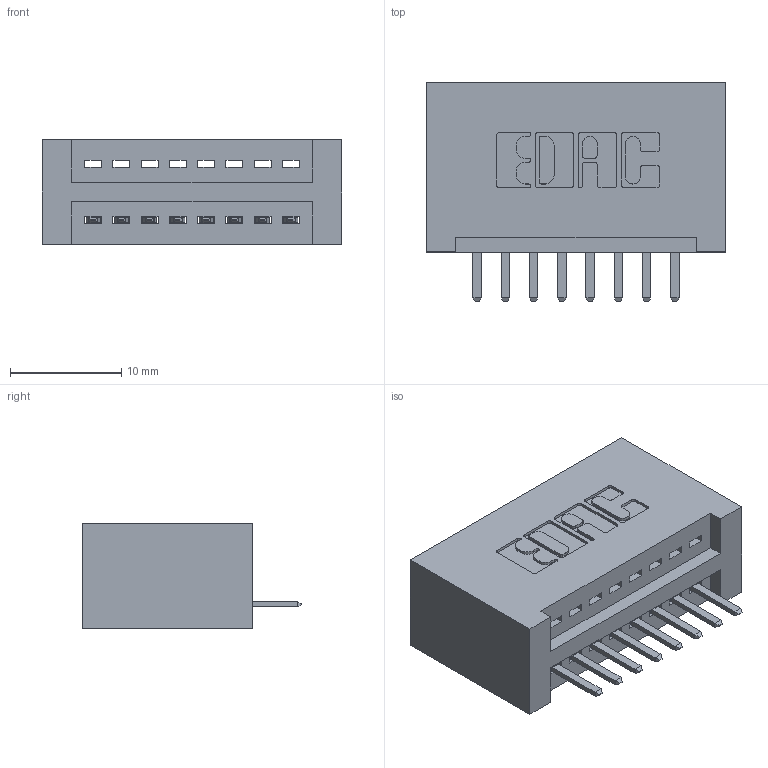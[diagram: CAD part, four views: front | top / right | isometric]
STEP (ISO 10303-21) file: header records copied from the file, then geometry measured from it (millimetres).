
FILE_DESCRIPTION (( 'STEP AP203' ), '1' );
FILE_NAME ('345-008-520-101.STEP', '2018-08-17T03:15:01', ( '' ), ( '' ), 'SwSTEP 2.0', 'SolidWorks 2016', '' );
FILE_SCHEMA (( 'CONFIG_CONTROL_DESIGN' ));
Length unit declared in the file: inch
Products named in the file (3): 345-008-520-101; 345 Part_No Mounting Lugs; 345-292-001_345-293-120
Assembly tree (9 placements, depth 2):
  345-008-520-101
    345 Part_No Mounting Lugs
    345-292-001_345-293-120  x8
Bounding box: 26.92 x 19.68 x 9.4 mm (x, y, z)
Volume: 2840.1 mm3; surface area: 3427 mm2
Topology: 9 solids, 9 shells, 614 faces, 1789 edges, 1170 vertices
Faces by surface type: plane 412, cylinder 202
Entity records: 10435 total; most frequent: CARTESIAN_POINT 1828, ORIENTED_EDGE 1758, DIRECTION 1627, EDGE_CURVE 879, LINE 719, VECTOR 719, VERTEX_POINT 582, AXIS2_PLACEMENT_3D 454
